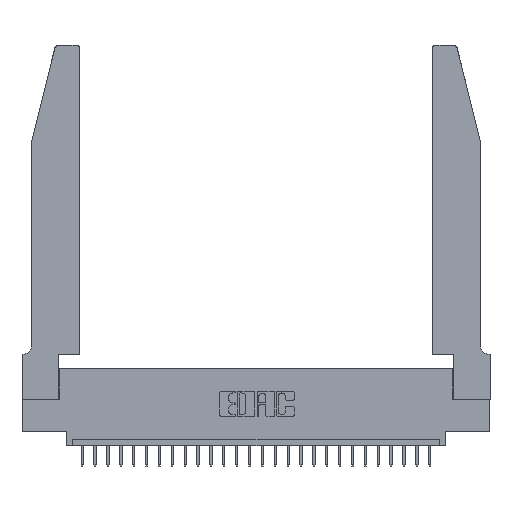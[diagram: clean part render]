
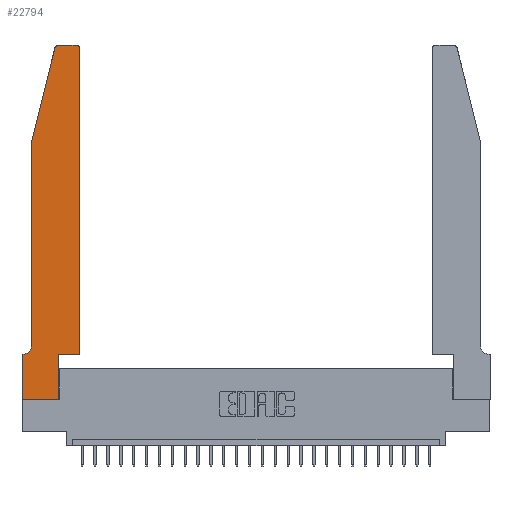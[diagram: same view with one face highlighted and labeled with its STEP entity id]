
A CAD part, top view. The second image highlights one B-rep face of the part: STEP entity #22794.
In plain terms, the highlighted planar face has unit normal (0, 0, 1).
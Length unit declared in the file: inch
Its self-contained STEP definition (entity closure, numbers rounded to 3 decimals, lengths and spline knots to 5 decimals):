
#92 = FACE_OUTER_BOUND ( 'NONE', #16521, .T. ) ;
#397 = EDGE_CURVE ( 'NONE', #6275, #8248, #17262, .T. ) ;
#467 = CARTESIAN_POINT ( 'NONE',  ( 0.0755, 2., 0.37 ) ) ;
#873 = ORIENTED_EDGE ( 'NONE', *, *, #4383, .T. ) ;
#897 = CARTESIAN_POINT ( 'NONE',  ( 0.0755, 2., 0.37 ) ) ;
#1318 = DIRECTION ( 'NONE',  ( -1., 0., 0. ) ) ;
#1391 = AXIS2_PLACEMENT_3D ( 'NONE', #8357, #6217, #21067 ) ;
#1439 = ORIENTED_EDGE ( 'NONE', *, *, #7730, .T. ) ;
#1772 = VECTOR ( 'NONE', #27766, 39.37008 ) ;
#1824 = VERTEX_POINT ( 'NONE', #18455 ) ;
#1950 = PLANE ( 'NONE',  #1391 ) ;
#2424 = DIRECTION ( 'NONE',  ( 1., 0., 0. ) ) ;
#2481 = CARTESIAN_POINT ( 'NONE',  ( 0.0755, 0.42, 0.37 ) ) ;
#3556 = CARTESIAN_POINT ( 'NONE',  ( 0., 0., 0.37 ) ) ;
#4040 = ORIENTED_EDGE ( 'NONE', *, *, #20440, .T. ) ;
#4284 = CARTESIAN_POINT ( 'NONE',  ( 0.25487, 2.72718, 0.37 ) ) ;
#4383 = EDGE_CURVE ( 'NONE', #5798, #16002, #19742, .T. ) ;
#4907 = LINE ( 'NONE', #17815, #14975 ) ;
#5127 = ORIENTED_EDGE ( 'NONE', *, *, #27898, .T. ) ;
#5525 = CARTESIAN_POINT ( 'NONE',  ( 0.0755, 0.35, 0.37 ) ) ;
#5565 = DIRECTION ( 'NONE',  ( 0., 1., 0. ) ) ;
#5798 = VERTEX_POINT ( 'NONE', #4284 ) ;
#5973 = CIRCLE ( 'NONE', #13811, 0.03 ) ;
#6217 = DIRECTION ( 'NONE',  ( 0., 0., 1. ) ) ;
#6275 = VERTEX_POINT ( 'NONE', #10432 ) ;
#6773 = VECTOR ( 'NONE', #19850, 39.37008 ) ;
#6792 = VECTOR ( 'NONE', #2424, 39.37008 ) ;
#6885 = VERTEX_POINT ( 'NONE', #3556 ) ;
#7668 = CARTESIAN_POINT ( 'NONE',  ( 0., 0.35, 0.37 ) ) ;
#7730 = EDGE_CURVE ( 'NONE', #23408, #22469, #9881, .T. ) ;
#7855 = VECTOR ( 'NONE', #1318, 39.37008 ) ;
#7996 = ORIENTED_EDGE ( 'NONE', *, *, #11476, .T. ) ;
#8146 = LINE ( 'NONE', #15515, #6792 ) ;
#8248 = VERTEX_POINT ( 'NONE', #18193 ) ;
#8357 = CARTESIAN_POINT ( 'NONE',  ( 0., 0.35, 0.37 ) ) ;
#8784 = ORIENTED_EDGE ( 'NONE', *, *, #397, .T. ) ;
#9881 = LINE ( 'NONE', #11770, #7855 ) ;
#10001 = LINE ( 'NONE', #5525, #10355 ) ;
#10181 = DIRECTION ( 'NONE',  ( 0., 0., 1. ) ) ;
#10343 = ORIENTED_EDGE ( 'NONE', *, *, #26173, .T. ) ;
#10355 = VECTOR ( 'NONE', #26843, 39.37008 ) ;
#10432 = CARTESIAN_POINT ( 'NONE',  ( 0.4505, 0.35, 0.37 ) ) ;
#10619 = ORIENTED_EDGE ( 'NONE', *, *, #15530, .T. ) ;
#10630 = DIRECTION ( 'NONE',  ( 1., 0., 0. ) ) ;
#11273 = ORIENTED_EDGE ( 'NONE', *, *, #13184, .T. ) ;
#11327 = VERTEX_POINT ( 'NONE', #2481 ) ;
#11476 = EDGE_CURVE ( 'NONE', #16408, #11488, #10001, .T. ) ;
#11488 = VERTEX_POINT ( 'NONE', #7668 ) ;
#11770 = CARTESIAN_POINT ( 'NONE',  ( 0.2605, 2.75, 0.37 ) ) ;
#11934 = DIRECTION ( 'NONE',  ( -0.239, -0.971, 0. ) ) ;
#13184 = EDGE_CURVE ( 'NONE', #22469, #5798, #5973, .T. ) ;
#13195 = EDGE_CURVE ( 'NONE', #8248, #23408, #16693, .T. ) ;
#13605 = DIRECTION ( 'NONE',  ( -1., 0., 0. ) ) ;
#13811 = AXIS2_PLACEMENT_3D ( 'NONE', #16482, #10181, #24865 ) ;
#13984 = CARTESIAN_POINT ( 'NONE',  ( 0.4505, 0.35, 0.37 ) ) ;
#14266 = CARTESIAN_POINT ( 'NONE',  ( 0.0055, 0.35, 0.37 ) ) ;
#14611 = CARTESIAN_POINT ( 'NONE',  ( 0., 0., 0.37 ) ) ;
#14778 = AXIS2_PLACEMENT_3D ( 'NONE', #24554, #26504, #13605 ) ;
#14975 = VECTOR ( 'NONE', #21941, 39.37008 ) ;
#14982 = CIRCLE ( 'NONE', #14778, 0.07 ) ;
#15455 = VECTOR ( 'NONE', #16763, 39.37008 ) ;
#15515 = CARTESIAN_POINT ( 'NONE',  ( 0.4505, 0.35, 0.37 ) ) ;
#15530 = EDGE_CURVE ( 'NONE', #1824, #23023, #15609, .T. ) ;
#15609 = LINE ( 'NONE', #19096, #1772 ) ;
#16002 = VERTEX_POINT ( 'NONE', #26462 ) ;
#16408 = VERTEX_POINT ( 'NONE', #14266 ) ;
#16482 = CARTESIAN_POINT ( 'NONE',  ( 0.284, 2.72, 0.37 ) ) ;
#16521 = EDGE_LOOP ( 'NONE', ( #1439, #11273, #873, #21204, #10343, #7996, #4040, #25656, #10619, #5127, #8784, #23165 ) ) ;
#16693 = CIRCLE ( 'NONE', #16700, 0.03 ) ;
#16700 = AXIS2_PLACEMENT_3D ( 'NONE', #25416, #21177, #10630 ) ;
#16763 = DIRECTION ( 'NONE',  ( 0., -1., 0. ) ) ;
#17262 = LINE ( 'NONE', #13984, #20985 ) ;
#17815 = CARTESIAN_POINT ( 'NONE',  ( 0., 0., 0.37 ) ) ;
#18193 = CARTESIAN_POINT ( 'NONE',  ( 0.4505, 2.72, 0.37 ) ) ;
#18455 = CARTESIAN_POINT ( 'NONE',  ( 0.2865, 0., 0.37 ) ) ;
#18777 = EDGE_CURVE ( 'NONE', #16002, #11327, #18887, .T. ) ;
#18887 = LINE ( 'NONE', #467, #6773 ) ;
#19096 = CARTESIAN_POINT ( 'NONE',  ( 0.2865, 0.35, 0.37 ) ) ;
#19742 = LINE ( 'NONE', #897, #26156 ) ;
#19850 = DIRECTION ( 'NONE',  ( 0., -1., 0. ) ) ;
#20440 = EDGE_CURVE ( 'NONE', #11488, #6885, #21503, .T. ) ;
#20985 = VECTOR ( 'NONE', #5565, 39.37008 ) ;
#21067 = DIRECTION ( 'NONE',  ( 1., 0., 0. ) ) ;
#21177 = DIRECTION ( 'NONE',  ( 0., 0., 1. ) ) ;
#21204 = ORIENTED_EDGE ( 'NONE', *, *, #18777, .T. ) ;
#21224 = CARTESIAN_POINT ( 'NONE',  ( 0.284, 2.75, 0.37 ) ) ;
#21503 = LINE ( 'NONE', #14611, #15455 ) ;
#21610 = CARTESIAN_POINT ( 'NONE',  ( 0.2865, 0.35, 0.37 ) ) ;
#21941 = DIRECTION ( 'NONE',  ( 1., 0., 0. ) ) ;
#22469 = VERTEX_POINT ( 'NONE', #21224 ) ;
#22794 = ADVANCED_FACE ( 'NONE', ( #92 ), #1950, .T. ) ;
#23023 = VERTEX_POINT ( 'NONE', #21610 ) ;
#23165 = ORIENTED_EDGE ( 'NONE', *, *, #13195, .T. ) ;
#23408 = VERTEX_POINT ( 'NONE', #23482 ) ;
#23482 = CARTESIAN_POINT ( 'NONE',  ( 0.4205, 2.75, 0.37 ) ) ;
#24554 = CARTESIAN_POINT ( 'NONE',  ( 0.0055, 0.42, 0.37 ) ) ;
#24865 = DIRECTION ( 'NONE',  ( 1., 0., 0. ) ) ;
#25329 = EDGE_CURVE ( 'NONE', #6885, #1824, #4907, .T. ) ;
#25416 = CARTESIAN_POINT ( 'NONE',  ( 0.4205, 2.72, 0.37 ) ) ;
#25656 = ORIENTED_EDGE ( 'NONE', *, *, #25329, .T. ) ;
#26156 = VECTOR ( 'NONE', #11934, 39.37008 ) ;
#26173 = EDGE_CURVE ( 'NONE', #11327, #16408, #14982, .T. ) ;
#26462 = CARTESIAN_POINT ( 'NONE',  ( 0.0755, 2., 0.37 ) ) ;
#26504 = DIRECTION ( 'NONE',  ( 0., 0., -1. ) ) ;
#26843 = DIRECTION ( 'NONE',  ( -1., 0., 0. ) ) ;
#27766 = DIRECTION ( 'NONE',  ( 0., 1., 0. ) ) ;
#27898 = EDGE_CURVE ( 'NONE', #23023, #6275, #8146, .T. ) ;
